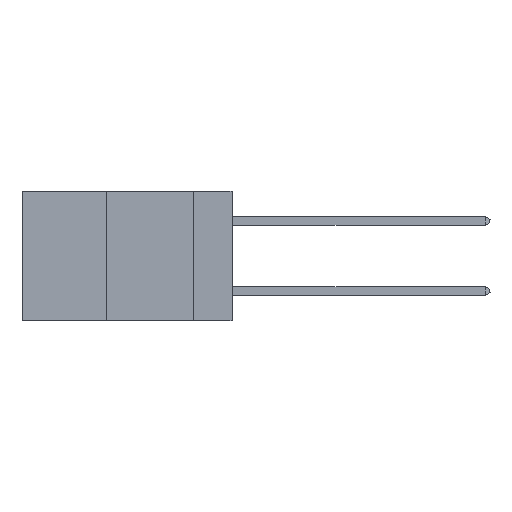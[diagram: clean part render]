
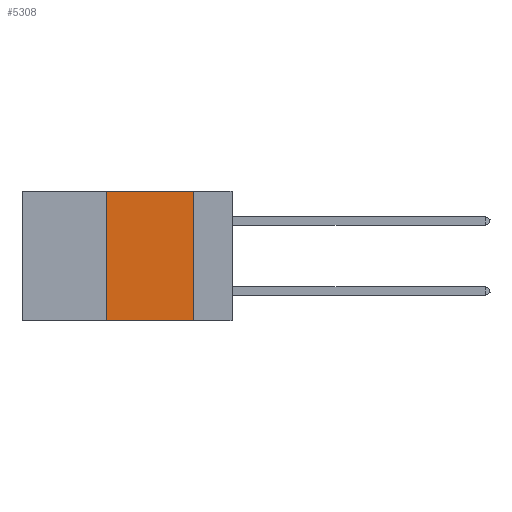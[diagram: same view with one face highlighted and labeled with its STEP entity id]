
A CAD part, left-side view. The second image highlights one B-rep face of the part: STEP entity #5308.
In plain terms, the highlighted planar face has unit normal (-1, 0, 0).
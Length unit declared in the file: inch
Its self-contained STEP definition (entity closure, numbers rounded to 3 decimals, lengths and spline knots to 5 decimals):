
#136 = CARTESIAN_POINT ( 'NONE',  ( 0., 0.6, 0. ) ) ;
#575 = EDGE_LOOP ( 'NONE', ( #31679, #18094, #11935, #19311 ) ) ;
#1003 = VERTEX_POINT ( 'NONE', #6248 ) ;
#3163 = VECTOR ( 'NONE', #41718, 39.37008 ) ;
#5308 = ADVANCED_FACE ( 'NONE', ( #41078 ), #21062, .F. ) ;
#5924 = VERTEX_POINT ( 'NONE', #20860 ) ;
#6248 = CARTESIAN_POINT ( 'NONE',  ( 0., 0.11, 0. ) ) ;
#6291 = CARTESIAN_POINT ( 'NONE',  ( 0., 0.36, -0.37 ) ) ;
#7429 = CARTESIAN_POINT ( 'NONE',  ( 0., 0.6, -0.37 ) ) ;
#10511 = AXIS2_PLACEMENT_3D ( 'NONE', #136, #32078, #24750 ) ;
#10603 = EDGE_CURVE ( 'NONE', #5924, #1003, #37625, .T. ) ;
#10933 = DIRECTION ( 'NONE',  ( 0., -1., 0. ) ) ;
#11935 = ORIENTED_EDGE ( 'NONE', *, *, #29479, .F. ) ;
#14804 = CARTESIAN_POINT ( 'NONE',  ( 0., 0.36, 0. ) ) ;
#17007 = LINE ( 'NONE', #7429, #23631 ) ;
#17339 = LINE ( 'NONE', #14804, #29381 ) ;
#18094 = ORIENTED_EDGE ( 'NONE', *, *, #10603, .F. ) ;
#18332 = DIRECTION ( 'NONE',  ( 0., 0., 1. ) ) ;
#19251 = CARTESIAN_POINT ( 'NONE',  ( 0., 0.11, 0. ) ) ;
#19311 = ORIENTED_EDGE ( 'NONE', *, *, #44707, .T. ) ;
#20860 = CARTESIAN_POINT ( 'NONE',  ( 0., 0.36, 0. ) ) ;
#21062 = PLANE ( 'NONE',  #10511 ) ;
#22618 = DIRECTION ( 'NONE',  ( 0., 0., -1. ) ) ;
#22696 = VERTEX_POINT ( 'NONE', #6291 ) ;
#23631 = VECTOR ( 'NONE', #10933, 39.37008 ) ;
#24750 = DIRECTION ( 'NONE',  ( 0., 0., -1. ) ) ;
#29381 = VECTOR ( 'NONE', #18332, 39.37008 ) ;
#29479 = EDGE_CURVE ( 'NONE', #22696, #5924, #17339, .T. ) ;
#31679 = ORIENTED_EDGE ( 'NONE', *, *, #41399, .F. ) ;
#32078 = DIRECTION ( 'NONE',  ( 1., 0., 0. ) ) ;
#32582 = LINE ( 'NONE', #19251, #36953 ) ;
#36953 = VECTOR ( 'NONE', #22618, 39.37008 ) ;
#37625 = LINE ( 'NONE', #41562, #3163 ) ;
#39954 = CARTESIAN_POINT ( 'NONE',  ( 0., 0.11, -0.37 ) ) ;
#41078 = FACE_OUTER_BOUND ( 'NONE', #575, .T. ) ;
#41399 = EDGE_CURVE ( 'NONE', #1003, #45034, #32582, .T. ) ;
#41562 = CARTESIAN_POINT ( 'NONE',  ( 0., 0.6, 0. ) ) ;
#41718 = DIRECTION ( 'NONE',  ( 0., -1., 0. ) ) ;
#44707 = EDGE_CURVE ( 'NONE', #22696, #45034, #17007, .T. ) ;
#45034 = VERTEX_POINT ( 'NONE', #39954 ) ;
